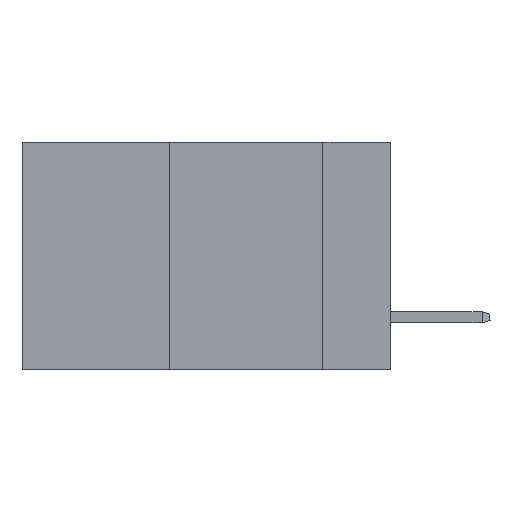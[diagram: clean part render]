
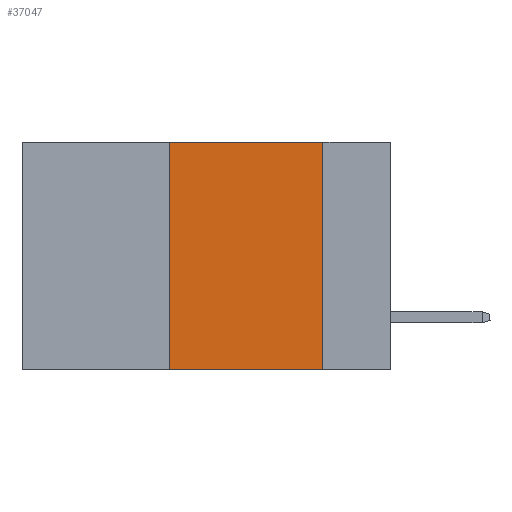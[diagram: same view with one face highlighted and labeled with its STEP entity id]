
A CAD part, left-side view. The second image highlights one B-rep face of the part: STEP entity #37047.
In plain terms, the highlighted planar face has unit normal (-1, 0, 0).
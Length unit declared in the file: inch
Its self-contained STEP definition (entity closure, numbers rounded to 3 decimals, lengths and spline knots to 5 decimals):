
#277 = EDGE_CURVE ( 'NONE', #30667, #37729, #5989, .T. ) ;
#1933 = EDGE_CURVE ( 'NONE', #30667, #26372, #16741, .T. ) ;
#1957 = ORIENTED_EDGE ( 'NONE', *, *, #277, .F. ) ;
#2699 = CARTESIAN_POINT ( 'NONE',  ( 0., 0.6, 0. ) ) ;
#3363 = FACE_OUTER_BOUND ( 'NONE', #10283, .T. ) ;
#3487 = VECTOR ( 'NONE', #14882, 39.37008 ) ;
#3686 = ORIENTED_EDGE ( 'NONE', *, *, #1933, .T. ) ;
#4069 = DIRECTION ( 'NONE',  ( 0., 0., -1. ) ) ;
#4914 = DIRECTION ( 'NONE',  ( 1., 0., 0. ) ) ;
#5173 = EDGE_CURVE ( 'NONE', #37729, #27040, #32614, .T. ) ;
#5989 = LINE ( 'NONE', #35788, #38180 ) ;
#7353 = CARTESIAN_POINT ( 'NONE',  ( 0., 0.11, 0. ) ) ;
#7638 = CARTESIAN_POINT ( 'NONE',  ( 0., 0.6, -0.37 ) ) ;
#10283 = EDGE_LOOP ( 'NONE', ( #34447, #11186, #1957, #3686 ) ) ;
#10699 = LINE ( 'NONE', #7353, #31534 ) ;
#11186 = ORIENTED_EDGE ( 'NONE', *, *, #5173, .F. ) ;
#12716 = EDGE_CURVE ( 'NONE', #27040, #26372, #10699, .T. ) ;
#14882 = DIRECTION ( 'NONE',  ( 0., -1., 0. ) ) ;
#16741 = LINE ( 'NONE', #7638, #24792 ) ;
#16776 = CARTESIAN_POINT ( 'NONE',  ( 0., 0.36, 0. ) ) ;
#16906 = AXIS2_PLACEMENT_3D ( 'NONE', #25692, #4914, #25830 ) ;
#20352 = CARTESIAN_POINT ( 'NONE',  ( 0., 0.11, 0. ) ) ;
#20462 = DIRECTION ( 'NONE',  ( 0., 0., 1. ) ) ;
#24792 = VECTOR ( 'NONE', #34750, 39.37008 ) ;
#24867 = CARTESIAN_POINT ( 'NONE',  ( 0., 0.36, -0.37 ) ) ;
#25692 = CARTESIAN_POINT ( 'NONE',  ( 0., 0.6, 0. ) ) ;
#25830 = DIRECTION ( 'NONE',  ( 0., 0., -1. ) ) ;
#26372 = VERTEX_POINT ( 'NONE', #32292 ) ;
#27040 = VERTEX_POINT ( 'NONE', #20352 ) ;
#30667 = VERTEX_POINT ( 'NONE', #24867 ) ;
#31534 = VECTOR ( 'NONE', #4069, 39.37008 ) ;
#31777 = PLANE ( 'NONE',  #16906 ) ;
#32292 = CARTESIAN_POINT ( 'NONE',  ( 0., 0.11, -0.37 ) ) ;
#32614 = LINE ( 'NONE', #2699, #3487 ) ;
#34447 = ORIENTED_EDGE ( 'NONE', *, *, #12716, .F. ) ;
#34750 = DIRECTION ( 'NONE',  ( 0., -1., 0. ) ) ;
#35788 = CARTESIAN_POINT ( 'NONE',  ( 0., 0.36, 0. ) ) ;
#37047 = ADVANCED_FACE ( 'NONE', ( #3363 ), #31777, .F. ) ;
#37729 = VERTEX_POINT ( 'NONE', #16776 ) ;
#38180 = VECTOR ( 'NONE', #20462, 39.37008 ) ;
